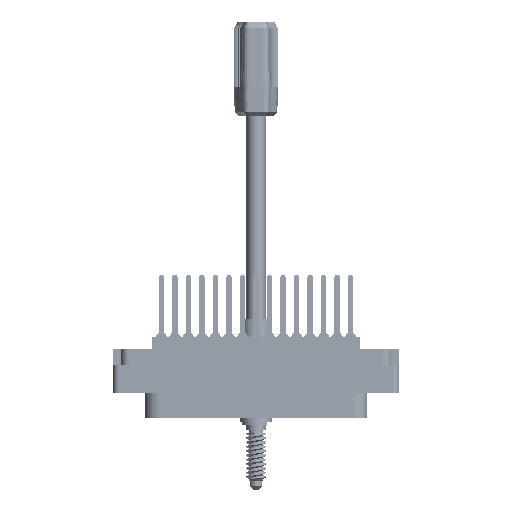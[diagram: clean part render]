
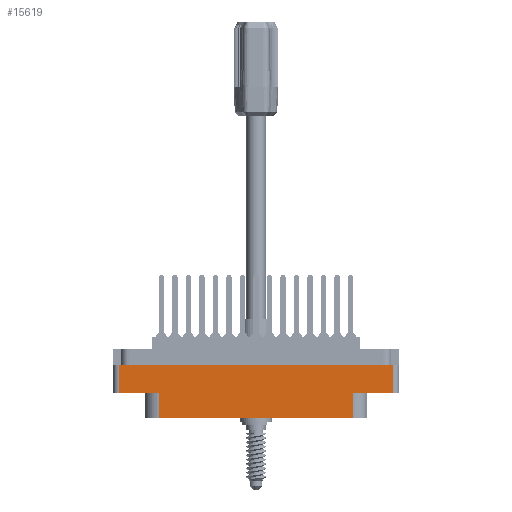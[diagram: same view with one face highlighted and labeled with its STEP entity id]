
A CAD part, front view. The second image highlights one B-rep face of the part: STEP entity #15619.
In plain terms, the highlighted planar face has unit normal (0, -1, 0).
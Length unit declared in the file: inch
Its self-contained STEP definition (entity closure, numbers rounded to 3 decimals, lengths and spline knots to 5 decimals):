
#1276 = ORIENTED_EDGE ( 'NONE', *, *, #86465, .T. ) ;
#3337 = CARTESIAN_POINT ( 'NONE',  ( 1.313, -0.7625, -0.274 ) ) ;
#3779 = ORIENTED_EDGE ( 'NONE', *, *, #14513, .T. ) ;
#4529 = ORIENTED_EDGE ( 'NONE', *, *, #75184, .F. ) ;
#9744 = LINE ( 'NONE', #42938, #33502 ) ;
#10515 = VECTOR ( 'NONE', #94974, 39.37008 ) ;
#13128 = LINE ( 'NONE', #70564, #51873 ) ;
#13842 = FACE_OUTER_BOUND ( 'NONE', #76533, .T. ) ;
#14513 = EDGE_CURVE ( 'NONE', #34186, #24833, #61796, .T. ) ;
#15619 = ADVANCED_FACE ( 'NONE', ( #13842 ), #68427, .T. ) ;
#16831 = CARTESIAN_POINT ( 'NONE',  ( -1.313, -0.7625, -0.78 ) ) ;
#19106 = EDGE_CURVE ( 'NONE', #38712, #34186, #79326, .T. ) ;
#24833 = VERTEX_POINT ( 'NONE', #55181 ) ;
#25005 = DIRECTION ( 'NONE',  ( 1., 0., 0. ) ) ;
#26776 = DIRECTION ( 'NONE',  ( 1., 0., 0. ) ) ;
#31201 = LINE ( 'NONE', #100156, #66114 ) ;
#32103 = ORIENTED_EDGE ( 'NONE', *, *, #88914, .F. ) ;
#33064 = DIRECTION ( 'NONE',  ( 1., 0., 0. ) ) ;
#33351 = VERTEX_POINT ( 'NONE', #94848 ) ;
#33502 = VECTOR ( 'NONE', #26776, 39.37008 ) ;
#33751 = CARTESIAN_POINT ( 'NONE',  ( -1.375, -0.7625, -0.78 ) ) ;
#34186 = VERTEX_POINT ( 'NONE', #55358 ) ;
#34750 = CARTESIAN_POINT ( 'NONE',  ( -0.9315, -0.7625, -0.54 ) ) ;
#35681 = CARTESIAN_POINT ( 'NONE',  ( -0.9315, -0.7625, -0.78 ) ) ;
#35698 = AXIS2_PLACEMENT_3D ( 'NONE', #69476, #37038, #92913 ) ;
#36260 = EDGE_CURVE ( 'NONE', #33351, #81208, #90638, .T. ) ;
#37038 = DIRECTION ( 'NONE',  ( 0., -1., 0. ) ) ;
#38712 = VERTEX_POINT ( 'NONE', #35681 ) ;
#38848 = EDGE_CURVE ( 'NONE', #98396, #39310, #102525, .T. ) ;
#39310 = VERTEX_POINT ( 'NONE', #3337 ) ;
#40172 = VERTEX_POINT ( 'NONE', #34750 ) ;
#41503 = DIRECTION ( 'NONE',  ( 0., 0., -1. ) ) ;
#42286 = ORIENTED_EDGE ( 'NONE', *, *, #85778, .T. ) ;
#42938 = CARTESIAN_POINT ( 'NONE',  ( 0., -0.7625, -0.54 ) ) ;
#46859 = DIRECTION ( 'NONE',  ( -1., 0., 0. ) ) ;
#46867 = VECTOR ( 'NONE', #33064, 39.37008 ) ;
#48398 = LINE ( 'NONE', #71745, #98331 ) ;
#51873 = VECTOR ( 'NONE', #46859, 39.37008 ) ;
#55181 = CARTESIAN_POINT ( 'NONE',  ( 0.9315, -0.7625, -0.54 ) ) ;
#55358 = CARTESIAN_POINT ( 'NONE',  ( 0.9315, -0.7625, -0.78 ) ) ;
#55635 = ORIENTED_EDGE ( 'NONE', *, *, #36260, .T. ) ;
#61796 = LINE ( 'NONE', #87664, #10515 ) ;
#66114 = VECTOR ( 'NONE', #76102, 39.37008 ) ;
#68427 = PLANE ( 'NONE',  #35698 ) ;
#69476 = CARTESIAN_POINT ( 'NONE',  ( -1.375, -0.7625, -0.78 ) ) ;
#70564 = CARTESIAN_POINT ( 'NONE',  ( 0., -0.7625, -0.54 ) ) ;
#71745 = CARTESIAN_POINT ( 'NONE',  ( 0., -0.7625, -0.274 ) ) ;
#74034 = CARTESIAN_POINT ( 'NONE',  ( -1.313, -0.7625, -0.54 ) ) ;
#75184 = EDGE_CURVE ( 'NONE', #33351, #39310, #48398, .T. ) ;
#76102 = DIRECTION ( 'NONE',  ( 0., 0., -1. ) ) ;
#76533 = EDGE_LOOP ( 'NONE', ( #4529, #55635, #1276, #42286, #93233, #3779, #32103, #85989 ) ) ;
#79326 = LINE ( 'NONE', #33751, #46867 ) ;
#81208 = VERTEX_POINT ( 'NONE', #74034 ) ;
#82621 = VECTOR ( 'NONE', #94171, 39.37008 ) ;
#85778 = EDGE_CURVE ( 'NONE', #40172, #38712, #31201, .T. ) ;
#85799 = CARTESIAN_POINT ( 'NONE',  ( 1.313, -0.7625, -0.78 ) ) ;
#85989 = ORIENTED_EDGE ( 'NONE', *, *, #38848, .T. ) ;
#86465 = EDGE_CURVE ( 'NONE', #81208, #40172, #9744, .T. ) ;
#87664 = CARTESIAN_POINT ( 'NONE',  ( 0.9315, -0.7625, -0.54 ) ) ;
#88914 = EDGE_CURVE ( 'NONE', #98396, #24833, #13128, .T. ) ;
#90638 = LINE ( 'NONE', #16831, #93153 ) ;
#92913 = DIRECTION ( 'NONE',  ( 0., 0., -1. ) ) ;
#93153 = VECTOR ( 'NONE', #41503, 39.37008 ) ;
#93233 = ORIENTED_EDGE ( 'NONE', *, *, #19106, .T. ) ;
#93453 = CARTESIAN_POINT ( 'NONE',  ( 1.313, -0.7625, -0.54 ) ) ;
#94171 = DIRECTION ( 'NONE',  ( 0., 0., 1. ) ) ;
#94848 = CARTESIAN_POINT ( 'NONE',  ( -1.313, -0.7625, -0.274 ) ) ;
#94974 = DIRECTION ( 'NONE',  ( 0., 0., 1. ) ) ;
#98331 = VECTOR ( 'NONE', #25005, 39.37008 ) ;
#98396 = VERTEX_POINT ( 'NONE', #93453 ) ;
#100156 = CARTESIAN_POINT ( 'NONE',  ( -0.9315, -0.7625, -0.78 ) ) ;
#102525 = LINE ( 'NONE', #85799, #82621 ) ;
